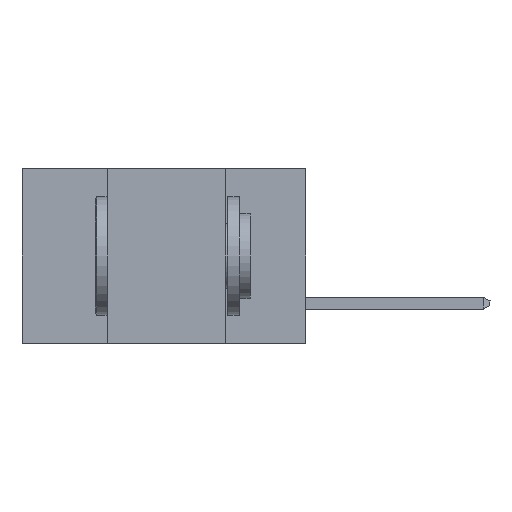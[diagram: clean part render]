
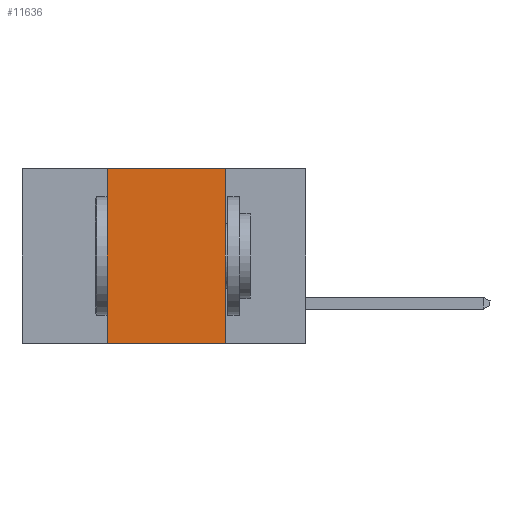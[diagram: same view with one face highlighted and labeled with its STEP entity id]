
A CAD part, left-side view. The second image highlights one B-rep face of the part: STEP entity #11636.
In plain terms, the highlighted planar face has unit normal (-1, 0, 0).
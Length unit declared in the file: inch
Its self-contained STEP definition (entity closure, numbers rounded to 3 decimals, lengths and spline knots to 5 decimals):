
#440 = CARTESIAN_POINT ( 'NONE',  ( 0., 0.6, 0. ) ) ;
#604 = DIRECTION ( 'NONE',  ( 0., -1., 0. ) ) ;
#1295 = VERTEX_POINT ( 'NONE', #3599 ) ;
#1480 = CARTESIAN_POINT ( 'NONE',  ( 0., 0.17, -0.37 ) ) ;
#1736 = DIRECTION ( 'NONE',  ( 0., -1., 0. ) ) ;
#1927 = AXIS2_PLACEMENT_3D ( 'NONE', #6933, #6816, #12127 ) ;
#2345 = VERTEX_POINT ( 'NONE', #5463 ) ;
#2863 = VECTOR ( 'NONE', #11637, 39.37008 ) ;
#2997 = FACE_OUTER_BOUND ( 'NONE', #8625, .T. ) ;
#3353 = EDGE_CURVE ( 'NONE', #2345, #11427, #15265, .T. ) ;
#3578 = ORIENTED_EDGE ( 'NONE', *, *, #3353, .T. ) ;
#3599 = CARTESIAN_POINT ( 'NONE',  ( 0., 0.42, 0. ) ) ;
#3792 = CARTESIAN_POINT ( 'NONE',  ( 0., 0.42, 0. ) ) ;
#4612 = ORIENTED_EDGE ( 'NONE', *, *, #5581, .F. ) ;
#5455 = EDGE_CURVE ( 'NONE', #2345, #1295, #12747, .T. ) ;
#5463 = CARTESIAN_POINT ( 'NONE',  ( 0., 0.42, -0.37 ) ) ;
#5517 = ORIENTED_EDGE ( 'NONE', *, *, #11043, .F. ) ;
#5581 = EDGE_CURVE ( 'NONE', #1295, #15074, #6265, .T. ) ;
#6265 = LINE ( 'NONE', #440, #10110 ) ;
#6816 = DIRECTION ( 'NONE',  ( 1., 0., 0. ) ) ;
#6933 = CARTESIAN_POINT ( 'NONE',  ( 0., 0.6, 0. ) ) ;
#8625 = EDGE_LOOP ( 'NONE', ( #5517, #4612, #14851, #3578 ) ) ;
#8926 = CARTESIAN_POINT ( 'NONE',  ( 0., 0.17, 0. ) ) ;
#8996 = VECTOR ( 'NONE', #604, 39.37008 ) ;
#9140 = DIRECTION ( 'NONE',  ( 0., 0., -1. ) ) ;
#9424 = PLANE ( 'NONE',  #1927 ) ;
#10110 = VECTOR ( 'NONE', #1736, 39.37008 ) ;
#11043 = EDGE_CURVE ( 'NONE', #15074, #11427, #13318, .T. ) ;
#11112 = CARTESIAN_POINT ( 'NONE',  ( 0., 0.6, -0.37 ) ) ;
#11427 = VERTEX_POINT ( 'NONE', #1480 ) ;
#11636 = ADVANCED_FACE ( 'NONE', ( #2997 ), #9424, .F. ) ;
#11637 = DIRECTION ( 'NONE',  ( 0., 0., 1. ) ) ;
#12127 = DIRECTION ( 'NONE',  ( 0., 0., -1. ) ) ;
#12747 = LINE ( 'NONE', #3792, #2863 ) ;
#13318 = LINE ( 'NONE', #8926, #16503 ) ;
#14105 = CARTESIAN_POINT ( 'NONE',  ( 0., 0.17, 0. ) ) ;
#14851 = ORIENTED_EDGE ( 'NONE', *, *, #5455, .F. ) ;
#15074 = VERTEX_POINT ( 'NONE', #14105 ) ;
#15265 = LINE ( 'NONE', #11112, #8996 ) ;
#16503 = VECTOR ( 'NONE', #9140, 39.37008 ) ;
